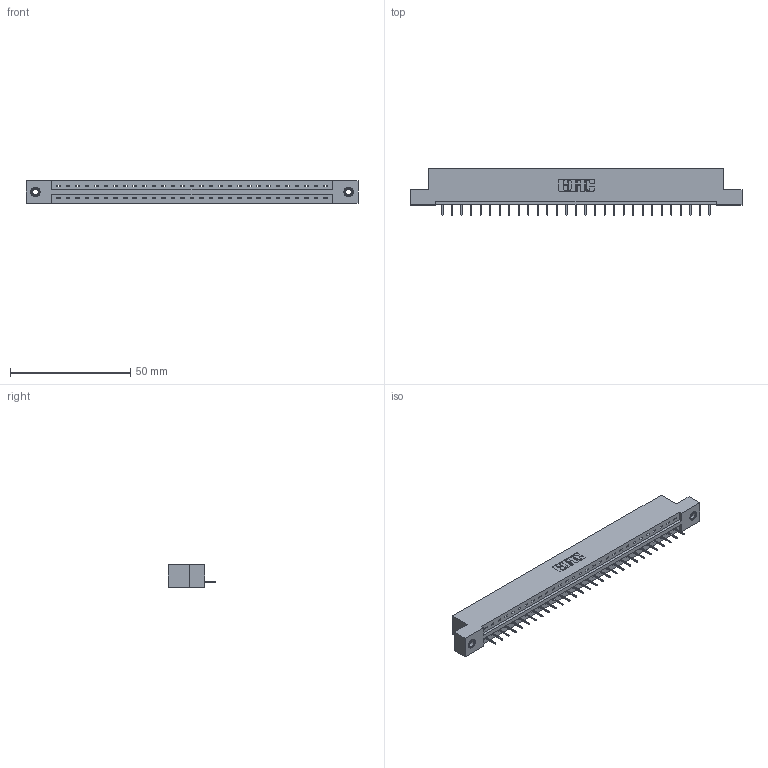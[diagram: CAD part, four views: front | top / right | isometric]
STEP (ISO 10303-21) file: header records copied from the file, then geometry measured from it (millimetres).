
FILE_DESCRIPTION (( 'STEP AP203' ), '1' );
FILE_NAME ('337-029-524-107.STEP', '2018-08-06T13:36:06', ( '' ), ( '' ), 'SwSTEP 2.0', 'SolidWorks 2016', '' );
FILE_SCHEMA (( 'CONFIG_CONTROL_DESIGN' ));
Length unit declared in the file: inch
Products named in the file (4): 345-292-001_345-293-124; 345-250-001_345-250-005-103; 337-029-524-107; 337 Part_Flush Mounting Lugs - 0.156 Dia-TI
Assembly tree (32 placements, depth 2):
  337-029-524-107
    337 Part_Flush Mounting Lugs - 0.156 Dia-TI
    345-292-001_345-293-124  x29
    345-250-001_345-250-005-103  x2
Bounding box: 137.92 x 19.69 x 9.4 mm (x, y, z)
Volume: 14043.9 mm3; surface area: 14078.4 mm2
Topology: 32 solids, 32 shells, 2088 faces, 6015 edges, 3886 vertices
Faces by surface type: plane 1610, cylinder 462, cone 12, torus 4
Entity records: 24498 total; most frequent: CARTESIAN_POINT 4244, ORIENTED_EDGE 4202, DIRECTION 3633, EDGE_CURVE 2101, VECTOR 1957, LINE 1957, VERTEX_POINT 1392, AXIS2_PLACEMENT_3D 838
